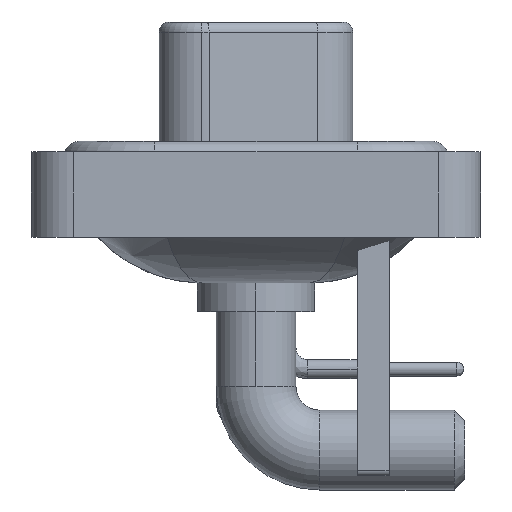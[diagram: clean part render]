
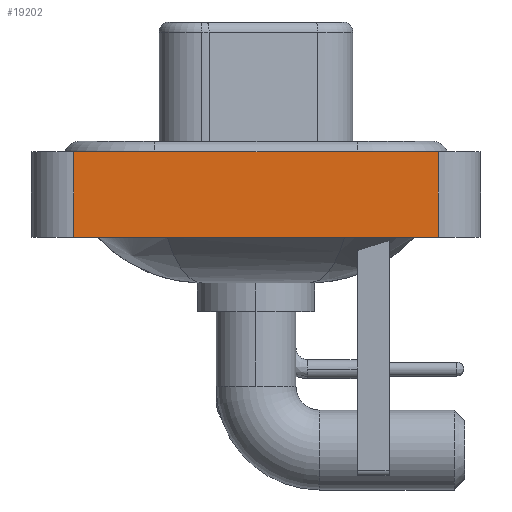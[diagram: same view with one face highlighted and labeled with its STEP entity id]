
A CAD part, left-side view. The second image highlights one B-rep face of the part: STEP entity #19202.
In plain terms, the highlighted planar face has unit normal (-1, 0, 0).
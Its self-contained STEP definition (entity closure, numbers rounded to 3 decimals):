
#50 = VERTEX_POINT ( 'NONE', #7631 ) ;
#183 = FACE_OUTER_BOUND ( 'NONE', #19979, .T. ) ;
#279 = VECTOR ( 'NONE', #18482, 1000. ) ;
#714 = LINE ( 'NONE', #4440, #8184 ) ;
#3500 = CARTESIAN_POINT ( 'NONE',  ( -7.3, 8.55, 0.4 ) ) ;
#3885 = DIRECTION ( 'NONE',  ( 0., -1., 0. ) ) ;
#4440 = CARTESIAN_POINT ( 'NONE',  ( -7.3, 8.55, -3.6 ) ) ;
#4967 = ORIENTED_EDGE ( 'NONE', *, *, #12242, .F. ) ;
#5302 = EDGE_CURVE ( 'NONE', #12607, #6185, #7327, .T. ) ;
#6185 = VERTEX_POINT ( 'NONE', #14640 ) ;
#7327 = LINE ( 'NONE', #7442, #9527 ) ;
#7442 = CARTESIAN_POINT ( 'NONE',  ( -7.3, -8.55, -3.6 ) ) ;
#7631 = CARTESIAN_POINT ( 'NONE',  ( -7.3, -8.55, 0.4 ) ) ;
#8184 = VECTOR ( 'NONE', #12247, 1000. ) ;
#9001 = VERTEX_POINT ( 'NONE', #3500 ) ;
#9527 = VECTOR ( 'NONE', #3885, 1000. ) ;
#10154 = DIRECTION ( 'NONE',  ( 0., 0., 1. ) ) ;
#10672 = LINE ( 'NONE', #24768, #279 ) ;
#11478 = ORIENTED_EDGE ( 'NONE', *, *, #5302, .T. ) ;
#12041 = EDGE_CURVE ( 'NONE', #12607, #9001, #714, .T. ) ;
#12242 = EDGE_CURVE ( 'NONE', #9001, #50, #19382, .T. ) ;
#12247 = DIRECTION ( 'NONE',  ( 0., 0., 1. ) ) ;
#12607 = VERTEX_POINT ( 'NONE', #16782 ) ;
#13476 = ORIENTED_EDGE ( 'NONE', *, *, #12041, .F. ) ;
#14122 = CARTESIAN_POINT ( 'NONE',  ( -7.3, -8.55, -3.6 ) ) ;
#14325 = ORIENTED_EDGE ( 'NONE', *, *, #23743, .T. ) ;
#14640 = CARTESIAN_POINT ( 'NONE',  ( -7.3, -8.55, -3.6 ) ) ;
#16746 = VECTOR ( 'NONE', #17306, 1000. ) ;
#16782 = CARTESIAN_POINT ( 'NONE',  ( -7.3, 8.55, -3.6 ) ) ;
#16923 = AXIS2_PLACEMENT_3D ( 'NONE', #14122, #21801, #10154 ) ;
#17306 = DIRECTION ( 'NONE',  ( 0., -1., 0. ) ) ;
#17820 = PLANE ( 'NONE',  #16923 ) ;
#18482 = DIRECTION ( 'NONE',  ( 0., 0., 1. ) ) ;
#19202 = ADVANCED_FACE ( 'NONE', ( #183 ), #17820, .T. ) ;
#19382 = LINE ( 'NONE', #19509, #16746 ) ;
#19509 = CARTESIAN_POINT ( 'NONE',  ( -7.3, -8.55, 0.4 ) ) ;
#19979 = EDGE_LOOP ( 'NONE', ( #14325, #4967, #13476, #11478 ) ) ;
#21801 = DIRECTION ( 'NONE',  ( -1., 0., 0. ) ) ;
#23743 = EDGE_CURVE ( 'NONE', #6185, #50, #10672, .T. ) ;
#24768 = CARTESIAN_POINT ( 'NONE',  ( -7.3, -8.55, -3.6 ) ) ;
